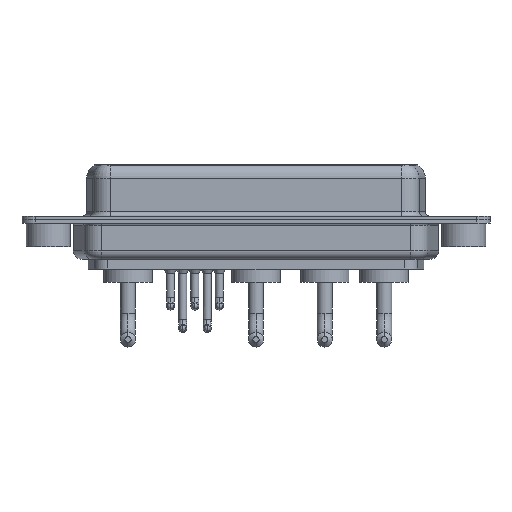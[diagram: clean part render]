
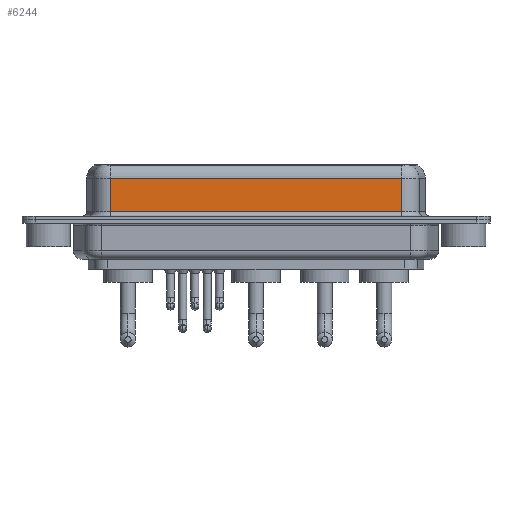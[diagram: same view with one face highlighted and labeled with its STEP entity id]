
A CAD part, front view. The second image highlights one B-rep face of the part: STEP entity #6244.
In plain terms, the highlighted planar face has unit normal (0, -1, 0).
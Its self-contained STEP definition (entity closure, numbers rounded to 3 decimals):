
#282 = CARTESIAN_POINT ( 'NONE',  ( 40.037, -3.95, 0.9 ) ) ;
#455 = VERTEX_POINT ( 'NONE', #11541 ) ;
#583 = CARTESIAN_POINT ( 'NONE',  ( 40.037, -3.95, 0.9 ) ) ;
#786 = ORIENTED_EDGE ( 'NONE', *, *, #3876, .T. ) ;
#987 = CARTESIAN_POINT ( 'NONE',  ( 40.037, -3.95, 4.65 ) ) ;
#1355 = VECTOR ( 'NONE', #8082, 1000. ) ;
#1418 = DIRECTION ( 'NONE',  ( 0., 0., -1. ) ) ;
#2180 = VECTOR ( 'NONE', #8958, 1000. ) ;
#2386 = LINE ( 'NONE', #2551, #14750 ) ;
#2551 = CARTESIAN_POINT ( 'NONE',  ( 40.037, -3.95, 6.4 ) ) ;
#2769 = DIRECTION ( 'NONE',  ( 0., 1., 0. ) ) ;
#2801 = EDGE_CURVE ( 'NONE', #7974, #455, #9045, .T. ) ;
#3392 = EDGE_CURVE ( 'NONE', #455, #17202, #7005, .T. ) ;
#3876 = EDGE_CURVE ( 'NONE', #17202, #12921, #4136, .T. ) ;
#4094 = FACE_OUTER_BOUND ( 'NONE', #16673, .T. ) ;
#4136 = LINE ( 'NONE', #282, #1355 ) ;
#4694 = DIRECTION ( 'NONE',  ( 0., 0., 1. ) ) ;
#4955 = EDGE_CURVE ( 'NONE', #7974, #12921, #2386, .T. ) ;
#6244 = ADVANCED_FACE ( 'NONE', ( #4094 ), #9437, .F. ) ;
#6412 = AXIS2_PLACEMENT_3D ( 'NONE', #14759, #2769, #4694 ) ;
#7005 = LINE ( 'NONE', #9627, #14204 ) ;
#7974 = VERTEX_POINT ( 'NONE', #9763 ) ;
#8082 = DIRECTION ( 'NONE',  ( 1., 0., 0. ) ) ;
#8958 = DIRECTION ( 'NONE',  ( -1., 0., 0. ) ) ;
#9045 = LINE ( 'NONE', #987, #2180 ) ;
#9437 = PLANE ( 'NONE',  #6412 ) ;
#9627 = CARTESIAN_POINT ( 'NONE',  ( 7.013, -3.95, 6.4 ) ) ;
#9763 = CARTESIAN_POINT ( 'NONE',  ( 40.037, -3.95, 4.65 ) ) ;
#11237 = ORIENTED_EDGE ( 'NONE', *, *, #2801, .T. ) ;
#11541 = CARTESIAN_POINT ( 'NONE',  ( 7.013, -3.95, 4.65 ) ) ;
#12505 = DIRECTION ( 'NONE',  ( 0., 0., -1. ) ) ;
#12625 = ORIENTED_EDGE ( 'NONE', *, *, #3392, .T. ) ;
#12921 = VERTEX_POINT ( 'NONE', #583 ) ;
#14204 = VECTOR ( 'NONE', #12505, 1000. ) ;
#14750 = VECTOR ( 'NONE', #1418, 1000. ) ;
#14759 = CARTESIAN_POINT ( 'NONE',  ( 40.037, -3.95, 6.4 ) ) ;
#15262 = CARTESIAN_POINT ( 'NONE',  ( 7.013, -3.95, 0.9 ) ) ;
#16673 = EDGE_LOOP ( 'NONE', ( #17286, #11237, #12625, #786 ) ) ;
#17202 = VERTEX_POINT ( 'NONE', #15262 ) ;
#17286 = ORIENTED_EDGE ( 'NONE', *, *, #4955, .F. ) ;
